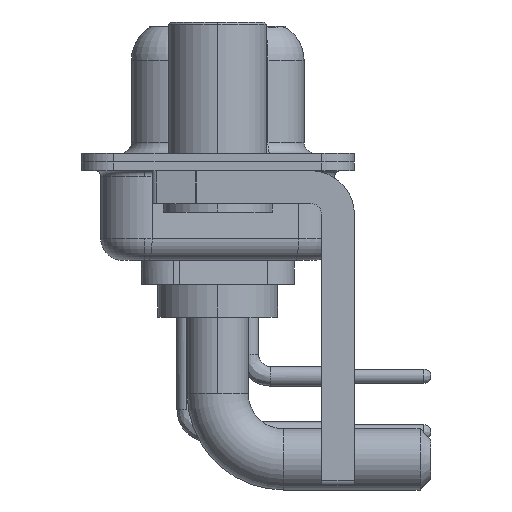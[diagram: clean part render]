
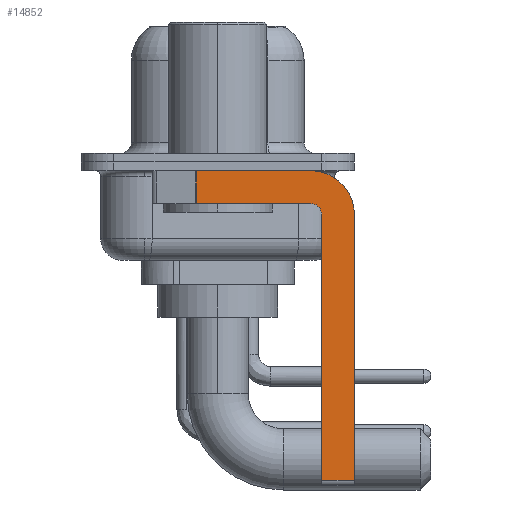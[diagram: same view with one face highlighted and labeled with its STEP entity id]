
A CAD part, left-side view. The second image highlights one B-rep face of the part: STEP entity #14852.
In plain terms, the highlighted planar face has unit normal (-1, 0, 0).
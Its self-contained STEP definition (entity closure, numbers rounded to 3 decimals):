
#28 = DIRECTION ( 'NONE',  ( 0., 0., -1. ) ) ;
#71 = VERTEX_POINT ( 'NONE', #5887 ) ;
#692 = LINE ( 'NONE', #6656, #14285 ) ;
#1016 = DIRECTION ( 'NONE',  ( 1., 0., 0. ) ) ;
#1687 = DIRECTION ( 'NONE',  ( -1., 0., 0. ) ) ;
#2185 = LINE ( 'NONE', #9750, #13775 ) ;
#2251 = CARTESIAN_POINT ( 'NONE',  ( -2.9, -4.25, -1.9 ) ) ;
#2446 = VECTOR ( 'NONE', #28, 1000. ) ;
#2544 = VERTEX_POINT ( 'NONE', #23254 ) ;
#2593 = EDGE_CURVE ( 'NONE', #3791, #3333, #5401, .T. ) ;
#3333 = VERTEX_POINT ( 'NONE', #2251 ) ;
#3540 = LINE ( 'NONE', #20402, #2446 ) ;
#3791 = VERTEX_POINT ( 'NONE', #8039 ) ;
#4310 = ORIENTED_EDGE ( 'NONE', *, *, #19840, .F. ) ;
#5194 = ORIENTED_EDGE ( 'NONE', *, *, #23129, .F. ) ;
#5372 = VECTOR ( 'NONE', #20987, 1000. ) ;
#5401 = CIRCLE ( 'NONE', #12510, 0.5 ) ;
#5429 = DIRECTION ( 'NONE',  ( 0., 0., 1. ) ) ;
#5707 = EDGE_CURVE ( 'NONE', #2544, #8948, #3540, .T. ) ;
#5872 = CARTESIAN_POINT ( 'NONE',  ( -2.9, -6.25, -2.4 ) ) ;
#5887 = CARTESIAN_POINT ( 'NONE',  ( -2.9, -6.25, -14.55 ) ) ;
#6656 = CARTESIAN_POINT ( 'NONE',  ( -2.9, 3., -0.4 ) ) ;
#7510 = VERTEX_POINT ( 'NONE', #16567 ) ;
#7529 = CARTESIAN_POINT ( 'NONE',  ( -2.9, -4.75, -14.8 ) ) ;
#7686 = DIRECTION ( 'NONE',  ( 0., -1., 0. ) ) ;
#8039 = CARTESIAN_POINT ( 'NONE',  ( -2.9, -4.75, -2.4 ) ) ;
#8948 = VERTEX_POINT ( 'NONE', #18193 ) ;
#9395 = LINE ( 'NONE', #7529, #18433 ) ;
#9750 = CARTESIAN_POINT ( 'NONE',  ( -2.9, -4.25, -14.55 ) ) ;
#9751 = CARTESIAN_POINT ( 'NONE',  ( -2.9, -6.25, -2.4 ) ) ;
#9774 = VERTEX_POINT ( 'NONE', #20333 ) ;
#9787 = VECTOR ( 'NONE', #11392, 1000. ) ;
#10299 = PLANE ( 'NONE',  #16973 ) ;
#10667 = DIRECTION ( 'NONE',  ( 1., 0., 0. ) ) ;
#11030 = EDGE_CURVE ( 'NONE', #7510, #3791, #9395, .T. ) ;
#11313 = ORIENTED_EDGE ( 'NONE', *, *, #23650, .T. ) ;
#11392 = DIRECTION ( 'NONE',  ( 0., 1., 0. ) ) ;
#11516 = LINE ( 'NONE', #15021, #9787 ) ;
#12172 = CIRCLE ( 'NONE', #18934, 2. ) ;
#12510 = AXIS2_PLACEMENT_3D ( 'NONE', #14625, #1687, #5429 ) ;
#13505 = ORIENTED_EDGE ( 'NONE', *, *, #11030, .F. ) ;
#13702 = ORIENTED_EDGE ( 'NONE', *, *, #2593, .F. ) ;
#13775 = VECTOR ( 'NONE', #20796, 1000. ) ;
#14285 = VECTOR ( 'NONE', #7686, 1000. ) ;
#14391 = EDGE_CURVE ( 'NONE', #9774, #17102, #12172, .T. ) ;
#14625 = CARTESIAN_POINT ( 'NONE',  ( -2.9, -4.25, -2.4 ) ) ;
#14755 = DIRECTION ( 'NONE',  ( 0., 0., 1. ) ) ;
#14852 = ADVANCED_FACE ( 'NONE', ( #21839 ), #10299, .F. ) ;
#15021 = CARTESIAN_POINT ( 'NONE',  ( -2.9, -4.25, -1.9 ) ) ;
#15339 = EDGE_CURVE ( 'NONE', #2544, #9774, #692, .T. ) ;
#15657 = ORIENTED_EDGE ( 'NONE', *, *, #15339, .F. ) ;
#15677 = LINE ( 'NONE', #5872, #5372 ) ;
#16038 = DIRECTION ( 'NONE',  ( 0., 0., -1. ) ) ;
#16567 = CARTESIAN_POINT ( 'NONE',  ( -2.9, -4.75, -14.55 ) ) ;
#16973 = AXIS2_PLACEMENT_3D ( 'NONE', #19979, #10667, #16038 ) ;
#17102 = VERTEX_POINT ( 'NONE', #9751 ) ;
#18183 = ORIENTED_EDGE ( 'NONE', *, *, #5707, .T. ) ;
#18193 = CARTESIAN_POINT ( 'NONE',  ( -2.9, 0.978, -1.9 ) ) ;
#18260 = DIRECTION ( 'NONE',  ( 0., 0., -1. ) ) ;
#18433 = VECTOR ( 'NONE', #14755, 1000. ) ;
#18934 = AXIS2_PLACEMENT_3D ( 'NONE', #20008, #1016, #18260 ) ;
#19207 = ORIENTED_EDGE ( 'NONE', *, *, #14391, .F. ) ;
#19840 = EDGE_CURVE ( 'NONE', #17102, #71, #15677, .T. ) ;
#19979 = CARTESIAN_POINT ( 'NONE',  ( -2.9, -4.25, -2.4 ) ) ;
#20008 = CARTESIAN_POINT ( 'NONE',  ( -2.9, -4.25, -2.4 ) ) ;
#20167 = EDGE_LOOP ( 'NONE', ( #15657, #18183, #5194, #13702, #13505, #11313, #4310, #19207 ) ) ;
#20333 = CARTESIAN_POINT ( 'NONE',  ( -2.9, -4.25, -0.4 ) ) ;
#20402 = CARTESIAN_POINT ( 'NONE',  ( -2.9, 0.978, -1.9 ) ) ;
#20796 = DIRECTION ( 'NONE',  ( 0., -1., 0. ) ) ;
#20987 = DIRECTION ( 'NONE',  ( 0., 0., -1. ) ) ;
#21839 = FACE_OUTER_BOUND ( 'NONE', #20167, .T. ) ;
#23129 = EDGE_CURVE ( 'NONE', #3333, #8948, #11516, .T. ) ;
#23254 = CARTESIAN_POINT ( 'NONE',  ( -2.9, 0.978, -0.4 ) ) ;
#23650 = EDGE_CURVE ( 'NONE', #7510, #71, #2185, .T. ) ;
